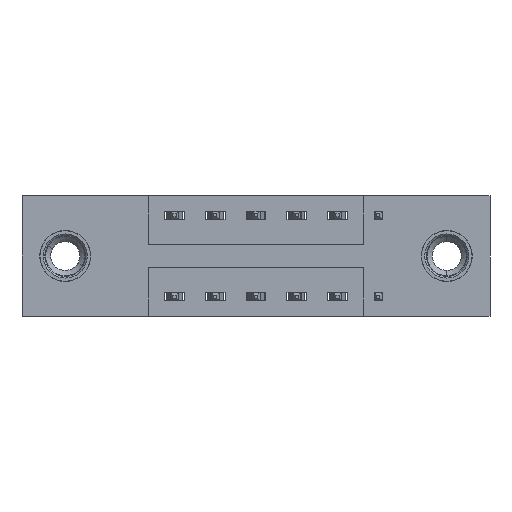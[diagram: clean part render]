
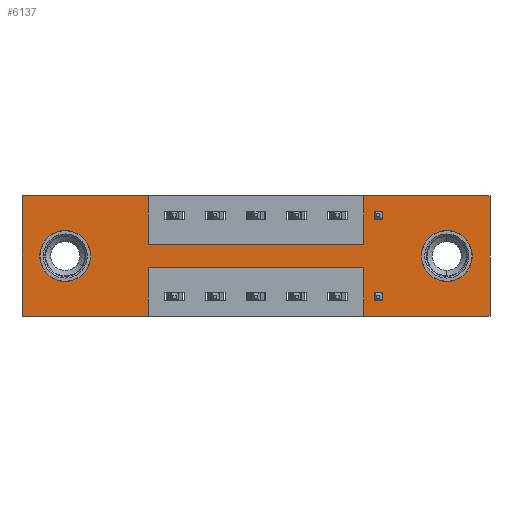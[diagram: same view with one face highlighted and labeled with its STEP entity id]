
A CAD part, front view. The second image highlights one B-rep face of the part: STEP entity #6137.
In plain terms, the highlighted planar face has unit normal (0, -1, 0).
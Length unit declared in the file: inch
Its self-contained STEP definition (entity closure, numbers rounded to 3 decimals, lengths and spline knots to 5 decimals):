
#96 = ORIENTED_EDGE ( 'NONE', *, *, #7327, .T. ) ;
#115 = CARTESIAN_POINT ( 'NONE',  ( 1.0475, 0., 0. ) ) ;
#189 = CARTESIAN_POINT ( 'NONE',  ( 1.0475, 0., -0.22 ) ) ;
#282 = VERTEX_POINT ( 'NONE', #1253 ) ;
#287 = AXIS2_PLACEMENT_3D ( 'NONE', #9078, #4061, #2446 ) ;
#333 = VECTOR ( 'NONE', #5156, 39.37008 ) ;
#364 = EDGE_CURVE ( 'NONE', #8003, #9440, #5921, .T. ) ;
#388 = CARTESIAN_POINT ( 'NONE',  ( 1.435, 0., 0. ) ) ;
#392 = ORIENTED_EDGE ( 'NONE', *, *, #6626, .F. ) ;
#458 = CIRCLE ( 'NONE', #5054, 0.078 ) ;
#707 = ORIENTED_EDGE ( 'NONE', *, *, #6522, .T. ) ;
#729 = EDGE_CURVE ( 'NONE', #6334, #4811, #4746, .T. ) ;
#755 = VECTOR ( 'NONE', #914, 39.37008 ) ;
#854 = ORIENTED_EDGE ( 'NONE', *, *, #1090, .T. ) ;
#887 = VERTEX_POINT ( 'NONE', #7473 ) ;
#914 = DIRECTION ( 'NONE',  ( 0., 0., 1. ) ) ;
#1078 = EDGE_LOOP ( 'NONE', ( #8640, #96 ) ) ;
#1090 = EDGE_CURVE ( 'NONE', #9243, #7855, #7046, .T. ) ;
#1172 = CARTESIAN_POINT ( 'NONE',  ( 0.3875, 0., -0.15 ) ) ;
#1184 = CARTESIAN_POINT ( 'NONE',  ( 0.1325, 0., -0.263 ) ) ;
#1196 = CARTESIAN_POINT ( 'NONE',  ( 1.0475, 0., -0.37 ) ) ;
#1226 = ORIENTED_EDGE ( 'NONE', *, *, #729, .F. ) ;
#1230 = DIRECTION ( 'NONE',  ( 0., 0., 1. ) ) ;
#1253 = CARTESIAN_POINT ( 'NONE',  ( 1.3025, 0., -0.107 ) ) ;
#1461 = CARTESIAN_POINT ( 'NONE',  ( 0.3875, 0., -0.37 ) ) ;
#1481 = CARTESIAN_POINT ( 'NONE',  ( 0.3875, 0., -0.37 ) ) ;
#1650 = CARTESIAN_POINT ( 'NONE',  ( 1.3025, 0., -0.185 ) ) ;
#1696 = CARTESIAN_POINT ( 'NONE',  ( 1.0475, 0., -0.15 ) ) ;
#1804 = VECTOR ( 'NONE', #9462, 39.37008 ) ;
#2079 = LINE ( 'NONE', #6644, #1804 ) ;
#2108 = VERTEX_POINT ( 'NONE', #6463 ) ;
#2195 = ORIENTED_EDGE ( 'NONE', *, *, #7907, .F. ) ;
#2276 = AXIS2_PLACEMENT_3D ( 'NONE', #6054, #9001, #3168 ) ;
#2286 = AXIS2_PLACEMENT_3D ( 'NONE', #4753, #7708, #2645 ) ;
#2312 = LINE ( 'NONE', #2351, #8750 ) ;
#2336 = ORIENTED_EDGE ( 'NONE', *, *, #5688, .F. ) ;
#2351 = CARTESIAN_POINT ( 'NONE',  ( 0., 0., -0.37 ) ) ;
#2379 = DIRECTION ( 'NONE',  ( 0., 0., -1. ) ) ;
#2446 = DIRECTION ( 'NONE',  ( 0., 0., -1. ) ) ;
#2451 = CARTESIAN_POINT ( 'NONE',  ( 0.3875, 0., -0.15 ) ) ;
#2468 = DIRECTION ( 'NONE',  ( 0., 1., 0. ) ) ;
#2645 = DIRECTION ( 'NONE',  ( 0., 0., 1. ) ) ;
#2795 = CARTESIAN_POINT ( 'NONE',  ( 0., 0., 0. ) ) ;
#2899 = VECTOR ( 'NONE', #2379, 39.37008 ) ;
#3077 = PLANE ( 'NONE',  #2276 ) ;
#3168 = DIRECTION ( 'NONE',  ( 0., 0., -1. ) ) ;
#3196 = CARTESIAN_POINT ( 'NONE',  ( 0.3875, 0., -0.22 ) ) ;
#3225 = VERTEX_POINT ( 'NONE', #189 ) ;
#3238 = VECTOR ( 'NONE', #5987, 39.37008 ) ;
#3240 = LINE ( 'NONE', #4870, #6126 ) ;
#3330 = EDGE_LOOP ( 'NONE', ( #6629, #2195, #3542, #6046, #2336, #9014, #4085, #5173, #1226, #7632, #392, #6681 ) ) ;
#3351 = CIRCLE ( 'NONE', #4106, 0.078 ) ;
#3530 = CARTESIAN_POINT ( 'NONE',  ( 0.1325, 0., -0.185 ) ) ;
#3542 = ORIENTED_EDGE ( 'NONE', *, *, #8500, .F. ) ;
#3624 = LINE ( 'NONE', #1481, #4933 ) ;
#3809 = CIRCLE ( 'NONE', #287, 0.078 ) ;
#4061 = DIRECTION ( 'NONE',  ( 0., 1., 0. ) ) ;
#4085 = ORIENTED_EDGE ( 'NONE', *, *, #364, .F. ) ;
#4106 = AXIS2_PLACEMENT_3D ( 'NONE', #1650, #2468, #7500 ) ;
#4567 = EDGE_CURVE ( 'NONE', #6686, #4900, #3624, .T. ) ;
#4607 = FACE_BOUND ( 'NONE', #7789, .T. ) ;
#4733 = CARTESIAN_POINT ( 'NONE',  ( 1.435, 0., 0. ) ) ;
#4746 = LINE ( 'NONE', #5514, #2899 ) ;
#4753 = CARTESIAN_POINT ( 'NONE',  ( 0.1325, 0., -0.185 ) ) ;
#4763 = CARTESIAN_POINT ( 'NONE',  ( 0.1325, 0., -0.107 ) ) ;
#4811 = VERTEX_POINT ( 'NONE', #2451 ) ;
#4870 = CARTESIAN_POINT ( 'NONE',  ( 0.3875, 0., -0.22 ) ) ;
#4887 = DIRECTION ( 'NONE',  ( 0., 1., 0. ) ) ;
#4900 = VERTEX_POINT ( 'NONE', #1461 ) ;
#4933 = VECTOR ( 'NONE', #8035, 39.37008 ) ;
#5054 = AXIS2_PLACEMENT_3D ( 'NONE', #3530, #4887, #1230 ) ;
#5156 = DIRECTION ( 'NONE',  ( 0., 0., 1. ) ) ;
#5172 = EDGE_CURVE ( 'NONE', #9440, #5238, #8052, .T. ) ;
#5173 = ORIENTED_EDGE ( 'NONE', *, *, #8997, .F. ) ;
#5238 = VERTEX_POINT ( 'NONE', #388 ) ;
#5252 = CARTESIAN_POINT ( 'NONE',  ( 0.3875, 0., 0. ) ) ;
#5454 = DIRECTION ( 'NONE',  ( 1., 0., 0. ) ) ;
#5458 = DIRECTION ( 'NONE',  ( -1., 0., 0. ) ) ;
#5514 = CARTESIAN_POINT ( 'NONE',  ( 0.3875, 0., 0. ) ) ;
#5638 = DIRECTION ( 'NONE',  ( 1., 0., 0. ) ) ;
#5688 = EDGE_CURVE ( 'NONE', #5238, #7709, #6847, .T. ) ;
#5841 = LINE ( 'NONE', #8801, #755 ) ;
#5921 = LINE ( 'NONE', #115, #333 ) ;
#5987 = DIRECTION ( 'NONE',  ( 0., 0., -1. ) ) ;
#6046 = ORIENTED_EDGE ( 'NONE', *, *, #7568, .F. ) ;
#6054 = CARTESIAN_POINT ( 'NONE',  ( 0., 0., -0.37 ) ) ;
#6126 = VECTOR ( 'NONE', #5458, 39.37008 ) ;
#6137 = ADVANCED_FACE ( 'NONE', ( #7487, #4607, #6736 ), #3077, .T. ) ;
#6334 = VERTEX_POINT ( 'NONE', #5252 ) ;
#6389 = LINE ( 'NONE', #2795, #8567 ) ;
#6463 = CARTESIAN_POINT ( 'NONE',  ( 1.0475, 0., -0.37 ) ) ;
#6496 = CARTESIAN_POINT ( 'NONE',  ( 1.435, 0., -0.37 ) ) ;
#6522 = EDGE_CURVE ( 'NONE', #7855, #9243, #458, .T. ) ;
#6626 = EDGE_CURVE ( 'NONE', #8712, #887, #5841, .T. ) ;
#6629 = ORIENTED_EDGE ( 'NONE', *, *, #4567, .F. ) ;
#6644 = CARTESIAN_POINT ( 'NONE',  ( 0., 0., -0.37 ) ) ;
#6681 = ORIENTED_EDGE ( 'NONE', *, *, #7059, .F. ) ;
#6686 = VERTEX_POINT ( 'NONE', #3196 ) ;
#6688 = DIRECTION ( 'NONE',  ( -1., 0., 0. ) ) ;
#6736 = FACE_OUTER_BOUND ( 'NONE', #3330, .T. ) ;
#6847 = LINE ( 'NONE', #4733, #3238 ) ;
#6937 = VERTEX_POINT ( 'NONE', #8400 ) ;
#7046 = CIRCLE ( 'NONE', #2286, 0.078 ) ;
#7059 = EDGE_CURVE ( 'NONE', #4900, #8712, #2079, .T. ) ;
#7076 = DIRECTION ( 'NONE',  ( 0., 0., 1. ) ) ;
#7123 = DIRECTION ( 'NONE',  ( 1., 0., 0. ) ) ;
#7327 = EDGE_CURVE ( 'NONE', #6937, #282, #3351, .T. ) ;
#7414 = CARTESIAN_POINT ( 'NONE',  ( 0., 0., -0.37 ) ) ;
#7473 = CARTESIAN_POINT ( 'NONE',  ( 0., 0., 0. ) ) ;
#7487 = FACE_BOUND ( 'NONE', #1078, .T. ) ;
#7500 = DIRECTION ( 'NONE',  ( 0., 0., -1. ) ) ;
#7568 = EDGE_CURVE ( 'NONE', #7709, #2108, #2312, .T. ) ;
#7632 = ORIENTED_EDGE ( 'NONE', *, *, #9357, .F. ) ;
#7708 = DIRECTION ( 'NONE',  ( 0., 1., 0. ) ) ;
#7709 = VERTEX_POINT ( 'NONE', #6496 ) ;
#7789 = EDGE_LOOP ( 'NONE', ( #854, #707 ) ) ;
#7825 = EDGE_CURVE ( 'NONE', #282, #6937, #3809, .T. ) ;
#7855 = VERTEX_POINT ( 'NONE', #1184 ) ;
#7907 = EDGE_CURVE ( 'NONE', #3225, #6686, #3240, .T. ) ;
#7920 = CARTESIAN_POINT ( 'NONE',  ( 0., 0., 0. ) ) ;
#7945 = VECTOR ( 'NONE', #7076, 39.37008 ) ;
#7952 = VECTOR ( 'NONE', #5454, 39.37008 ) ;
#8003 = VERTEX_POINT ( 'NONE', #1696 ) ;
#8035 = DIRECTION ( 'NONE',  ( 0., 0., -1. ) ) ;
#8052 = LINE ( 'NONE', #7920, #9261 ) ;
#8400 = CARTESIAN_POINT ( 'NONE',  ( 1.3025, 0., -0.263 ) ) ;
#8500 = EDGE_CURVE ( 'NONE', #2108, #3225, #9293, .T. ) ;
#8529 = CARTESIAN_POINT ( 'NONE',  ( 1.0475, 0., 0. ) ) ;
#8567 = VECTOR ( 'NONE', #7123, 39.37008 ) ;
#8640 = ORIENTED_EDGE ( 'NONE', *, *, #7825, .T. ) ;
#8712 = VERTEX_POINT ( 'NONE', #7414 ) ;
#8750 = VECTOR ( 'NONE', #6688, 39.37008 ) ;
#8801 = CARTESIAN_POINT ( 'NONE',  ( 0., 0., 0. ) ) ;
#8997 = EDGE_CURVE ( 'NONE', #4811, #8003, #9317, .T. ) ;
#9001 = DIRECTION ( 'NONE',  ( 0., -1., 0. ) ) ;
#9014 = ORIENTED_EDGE ( 'NONE', *, *, #5172, .F. ) ;
#9078 = CARTESIAN_POINT ( 'NONE',  ( 1.3025, 0., -0.185 ) ) ;
#9243 = VERTEX_POINT ( 'NONE', #4763 ) ;
#9261 = VECTOR ( 'NONE', #5638, 39.37008 ) ;
#9293 = LINE ( 'NONE', #1196, #7945 ) ;
#9317 = LINE ( 'NONE', #1172, #7952 ) ;
#9357 = EDGE_CURVE ( 'NONE', #887, #6334, #6389, .T. ) ;
#9440 = VERTEX_POINT ( 'NONE', #8529 ) ;
#9462 = DIRECTION ( 'NONE',  ( -1., 0., 0. ) ) ;
